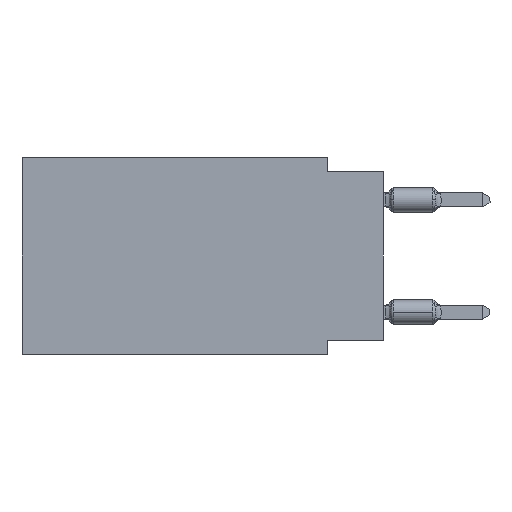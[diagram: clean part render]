
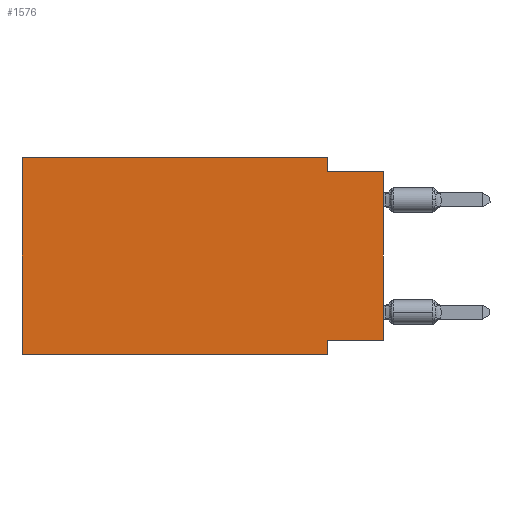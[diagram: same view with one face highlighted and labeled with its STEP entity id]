
A CAD part, left-side view. The second image highlights one B-rep face of the part: STEP entity #1576.
In plain terms, the highlighted planar face has unit normal (-1, 0, 0).
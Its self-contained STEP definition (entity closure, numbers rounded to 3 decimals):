
#160 = CARTESIAN_POINT ( 'NONE',  ( 0., 2.54, -8.89 ) ) ;
#480 = CARTESIAN_POINT ( 'NONE',  ( 0., 0., -0.635 ) ) ;
#642 = VERTEX_POINT ( 'NONE', #684 ) ;
#684 = CARTESIAN_POINT ( 'NONE',  ( 0., 0., -0.635 ) ) ;
#907 = LINE ( 'NONE', #11664, #14644 ) ;
#989 = DIRECTION ( 'NONE',  ( 0., 0., 1. ) ) ;
#992 = VERTEX_POINT ( 'NONE', #11754 ) ;
#1361 = CARTESIAN_POINT ( 'NONE',  ( 0., 16.383, -8.89 ) ) ;
#1576 = ADVANCED_FACE ( 'NONE', ( #3636 ), #10639, .F. ) ;
#1669 = VECTOR ( 'NONE', #9551, 1000. ) ;
#1860 = CARTESIAN_POINT ( 'NONE',  ( 0., 2.54, -0.635 ) ) ;
#2663 = EDGE_LOOP ( 'NONE', ( #9289, #10505, #8515, #13443, #8885, #7557, #7764, #9013 ) ) ;
#3589 = EDGE_CURVE ( 'NONE', #5676, #12910, #907, .T. ) ;
#3636 = FACE_OUTER_BOUND ( 'NONE', #2663, .T. ) ;
#3753 = VERTEX_POINT ( 'NONE', #6224 ) ;
#4048 = EDGE_CURVE ( 'NONE', #992, #11951, #14691, .T. ) ;
#4330 = DIRECTION ( 'NONE',  ( 0., -1., 0. ) ) ;
#4401 = VECTOR ( 'NONE', #14391, 1000. ) ;
#4595 = DIRECTION ( 'NONE',  ( 0., 0., 1. ) ) ;
#4986 = EDGE_CURVE ( 'NONE', #8850, #642, #15200, .T. ) ;
#5407 = DIRECTION ( 'NONE',  ( 0., 0., -1. ) ) ;
#5599 = EDGE_CURVE ( 'NONE', #12910, #992, #14844, .T. ) ;
#5676 = VERTEX_POINT ( 'NONE', #11769 ) ;
#6224 = CARTESIAN_POINT ( 'NONE',  ( 0., 2.54, -8.255 ) ) ;
#6269 = DIRECTION ( 'NONE',  ( 0., -1., 0. ) ) ;
#6387 = CARTESIAN_POINT ( 'NONE',  ( 0., 2.54, -8.89 ) ) ;
#6527 = CARTESIAN_POINT ( 'NONE',  ( 0., 16.383, 0. ) ) ;
#6973 = CARTESIAN_POINT ( 'NONE',  ( 0., 0., -8.255 ) ) ;
#7557 = ORIENTED_EDGE ( 'NONE', *, *, #11317, .T. ) ;
#7764 = ORIENTED_EDGE ( 'NONE', *, *, #10495, .F. ) ;
#7871 = CARTESIAN_POINT ( 'NONE',  ( 0., 16.383, 0. ) ) ;
#8515 = ORIENTED_EDGE ( 'NONE', *, *, #4048, .F. ) ;
#8622 = AXIS2_PLACEMENT_3D ( 'NONE', #14077, #10558, #9186 ) ;
#8850 = VERTEX_POINT ( 'NONE', #6973 ) ;
#8885 = ORIENTED_EDGE ( 'NONE', *, *, #3589, .F. ) ;
#8997 = EDGE_CURVE ( 'NONE', #8850, #3753, #12240, .T. ) ;
#9013 = ORIENTED_EDGE ( 'NONE', *, *, #8997, .F. ) ;
#9086 = EDGE_CURVE ( 'NONE', #11951, #642, #9713, .T. ) ;
#9186 = DIRECTION ( 'NONE',  ( 0., 0., -1. ) ) ;
#9289 = ORIENTED_EDGE ( 'NONE', *, *, #4986, .T. ) ;
#9551 = DIRECTION ( 'NONE',  ( 0., 0., -1. ) ) ;
#9713 = LINE ( 'NONE', #480, #14682 ) ;
#10264 = VECTOR ( 'NONE', #4595, 1000. ) ;
#10495 = EDGE_CURVE ( 'NONE', #3753, #14013, #13075, .T. ) ;
#10505 = ORIENTED_EDGE ( 'NONE', *, *, #9086, .F. ) ;
#10558 = DIRECTION ( 'NONE',  ( 1., 0., 0. ) ) ;
#10639 = PLANE ( 'NONE',  #8622 ) ;
#11162 = CARTESIAN_POINT ( 'NONE',  ( 0., 0., -8.255 ) ) ;
#11317 = EDGE_CURVE ( 'NONE', #5676, #14013, #14114, .T. ) ;
#11664 = CARTESIAN_POINT ( 'NONE',  ( 0., 16.383, 0. ) ) ;
#11754 = CARTESIAN_POINT ( 'NONE',  ( 0., 2.54, 0. ) ) ;
#11769 = CARTESIAN_POINT ( 'NONE',  ( 0., 16.383, -8.89 ) ) ;
#11951 = VERTEX_POINT ( 'NONE', #1860 ) ;
#12186 = VECTOR ( 'NONE', #5407, 1000. ) ;
#12240 = LINE ( 'NONE', #11162, #4401 ) ;
#12906 = VECTOR ( 'NONE', #14042, 1000. ) ;
#12910 = VERTEX_POINT ( 'NONE', #6527 ) ;
#13075 = LINE ( 'NONE', #160, #1669 ) ;
#13443 = ORIENTED_EDGE ( 'NONE', *, *, #5599, .F. ) ;
#13686 = CARTESIAN_POINT ( 'NONE',  ( 0., 2.54, 0. ) ) ;
#13868 = CARTESIAN_POINT ( 'NONE',  ( 0., 0., 0. ) ) ;
#14013 = VERTEX_POINT ( 'NONE', #6387 ) ;
#14042 = DIRECTION ( 'NONE',  ( 0., -1., 0. ) ) ;
#14077 = CARTESIAN_POINT ( 'NONE',  ( 0., 16.383, 0. ) ) ;
#14114 = LINE ( 'NONE', #1361, #12906 ) ;
#14391 = DIRECTION ( 'NONE',  ( 0., 1., 0. ) ) ;
#14605 = VECTOR ( 'NONE', #4330, 1000. ) ;
#14644 = VECTOR ( 'NONE', #989, 1000. ) ;
#14682 = VECTOR ( 'NONE', #6269, 1000. ) ;
#14691 = LINE ( 'NONE', #13686, #12186 ) ;
#14844 = LINE ( 'NONE', #7871, #14605 ) ;
#15200 = LINE ( 'NONE', #13868, #10264 ) ;
